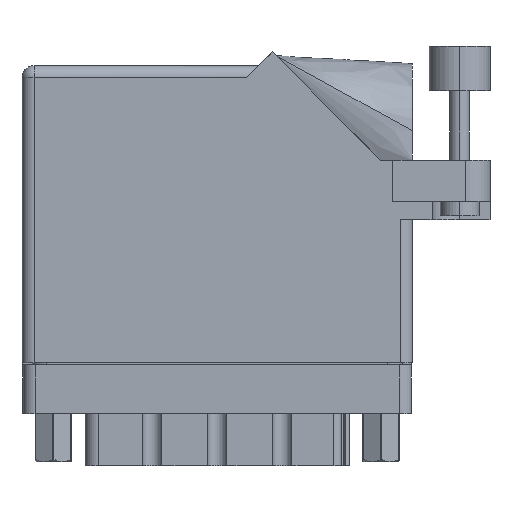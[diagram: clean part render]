
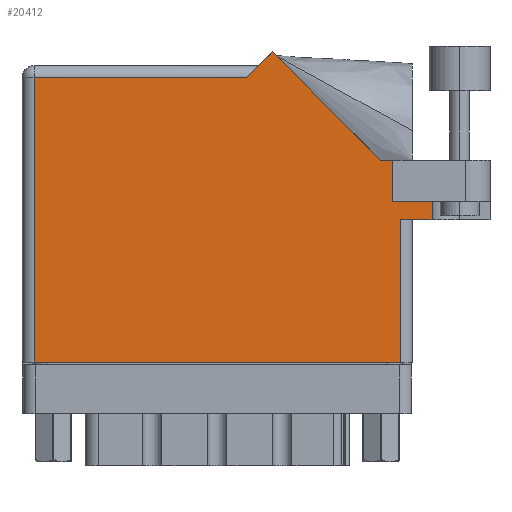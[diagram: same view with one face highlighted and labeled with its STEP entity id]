
A CAD part, front view. The second image highlights one B-rep face of the part: STEP entity #20412.
In plain terms, the highlighted face is planar.
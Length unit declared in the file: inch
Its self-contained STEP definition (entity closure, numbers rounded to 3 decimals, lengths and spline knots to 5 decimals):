
#869 = VECTOR ( 'NONE', #41921, 39.37008 ) ;
#1290 = VERTEX_POINT ( 'NONE', #13275 ) ;
#1875 = VERTEX_POINT ( 'NONE', #25170 ) ;
#2130 = VERTEX_POINT ( 'NONE', #23247 ) ;
#2452 = CARTESIAN_POINT ( 'NONE',  ( 0.062, 0., 0. ) ) ;
#2552 = CARTESIAN_POINT ( 'NONE',  ( 0.062, 1.468, 0. ) ) ;
#2928 = DIRECTION ( 'NONE',  ( -0.707, -0.707, 0. ) ) ;
#4628 = VECTOR ( 'NONE', #13545, 39.37008 ) ;
#5294 = CARTESIAN_POINT ( 'NONE',  ( 1.91, 0.831, 0. ) ) ;
#5372 = LINE ( 'NONE', #5294, #10856 ) ;
#6090 = ORIENTED_EDGE ( 'NONE', *, *, #49748, .T. ) ;
#7015 = CARTESIAN_POINT ( 'NONE',  ( 1.217, 1.53, 0. ) ) ;
#7782 = LINE ( 'NONE', #17917, #24767 ) ;
#8381 = CARTESIAN_POINT ( 'NONE',  ( 1.948, 0., 0. ) ) ;
#9344 = LINE ( 'NONE', #27450, #49462 ) ;
#9447 = DIRECTION ( 'NONE',  ( -1., 0., 0. ) ) ;
#10003 = VECTOR ( 'NONE', #2928, 39.37008 ) ;
#10309 = EDGE_CURVE ( 'NONE', #1290, #27184, #21557, .T. ) ;
#10856 = VECTOR ( 'NONE', #32533, 39.37008 ) ;
#10912 = ORIENTED_EDGE ( 'NONE', *, *, #29694, .T. ) ;
#11082 = VECTOR ( 'NONE', #19312, 39.37008 ) ;
#11657 = DIRECTION ( 'NONE',  ( 0., 1., 0. ) ) ;
#11774 = ORIENTED_EDGE ( 'NONE', *, *, #29884, .T. ) ;
#11809 = VERTEX_POINT ( 'NONE', #26147 ) ;
#13275 = CARTESIAN_POINT ( 'NONE',  ( 1.28771, 1.60071, 0. ) ) ;
#13545 = DIRECTION ( 'NONE',  ( 0., -1., 0. ) ) ;
#13706 = CARTESIAN_POINT ( 'NONE',  ( 1.91, 0.831, 0. ) ) ;
#13804 = VERTEX_POINT ( 'NONE', #38779 ) ;
#15364 = EDGE_CURVE ( 'NONE', #43490, #1875, #5372, .T. ) ;
#16979 = EDGE_LOOP ( 'NONE', ( #19858, #11774, #18190, #32483, #29464, #48066, #10912, #41270, #43193, #6090, #35443 ) ) ;
#17917 = CARTESIAN_POINT ( 'NONE',  ( 0., 1.468, 0. ) ) ;
#18190 = ORIENTED_EDGE ( 'NONE', *, *, #46316, .T. ) ;
#19312 = DIRECTION ( 'NONE',  ( 0., -1., 0. ) ) ;
#19858 = ORIENTED_EDGE ( 'NONE', *, *, #24635, .T. ) ;
#20273 = VERTEX_POINT ( 'NONE', #27319 ) ;
#20412 = ADVANCED_FACE ( 'NONE', ( #48146 ), #47375, .F. ) ;
#20716 = VECTOR ( 'NONE', #22096, 39.37008 ) ;
#21557 = LINE ( 'NONE', #7015, #10003 ) ;
#22037 = CARTESIAN_POINT ( 'NONE',  ( 0., 0., 0. ) ) ;
#22096 = DIRECTION ( 'NONE',  ( -1., 0., 0. ) ) ;
#23247 = CARTESIAN_POINT ( 'NONE',  ( 1.84442, 1.044, 0. ) ) ;
#24066 = DIRECTION ( 'NONE',  ( 0., 0., -1. ) ) ;
#24635 = EDGE_CURVE ( 'NONE', #40682, #27540, #41026, .T. ) ;
#24767 = VECTOR ( 'NONE', #9447, 39.37008 ) ;
#24804 = CARTESIAN_POINT ( 'NONE',  ( 1.84442, 1.044, 0. ) ) ;
#24969 = DIRECTION ( 'NONE',  ( -0.707, 0.707, 0. ) ) ;
#25170 = CARTESIAN_POINT ( 'NONE',  ( 2.1115, 0.831, 0. ) ) ;
#25389 = EDGE_CURVE ( 'NONE', #2130, #1290, #39785, .T. ) ;
#25586 = EDGE_CURVE ( 'NONE', #43490, #13804, #9344, .T. ) ;
#26147 = CARTESIAN_POINT ( 'NONE',  ( 1.948, 0.737, 0. ) ) ;
#26801 = LINE ( 'NONE', #37617, #20716 ) ;
#27184 = VERTEX_POINT ( 'NONE', #30011 ) ;
#27319 = CARTESIAN_POINT ( 'NONE',  ( 2.1115, 0.737, 0. ) ) ;
#27450 = CARTESIAN_POINT ( 'NONE',  ( 1.91, 0.831, 0. ) ) ;
#27540 = VERTEX_POINT ( 'NONE', #8381 ) ;
#29464 = ORIENTED_EDGE ( 'NONE', *, *, #15364, .F. ) ;
#29694 = EDGE_CURVE ( 'NONE', #13804, #2130, #26801, .T. ) ;
#29884 = EDGE_CURVE ( 'NONE', #27540, #11809, #43830, .T. ) ;
#30011 = CARTESIAN_POINT ( 'NONE',  ( 1.155, 1.468, 0. ) ) ;
#30642 = AXIS2_PLACEMENT_3D ( 'NONE', #35525, #24066, #47543 ) ;
#32483 = ORIENTED_EDGE ( 'NONE', *, *, #47893, .F. ) ;
#32533 = DIRECTION ( 'NONE',  ( 1., 0., 0. ) ) ;
#32699 = DIRECTION ( 'NONE',  ( 1., 0., 0. ) ) ;
#33525 = VECTOR ( 'NONE', #50132, 39.37008 ) ;
#34245 = LINE ( 'NONE', #2452, #11082 ) ;
#34546 = CARTESIAN_POINT ( 'NONE',  ( 1.948, 0.737, 0. ) ) ;
#35443 = ORIENTED_EDGE ( 'NONE', *, *, #43655, .T. ) ;
#35525 = CARTESIAN_POINT ( 'NONE',  ( 0., 1.53, 0. ) ) ;
#37613 = VECTOR ( 'NONE', #32699, 39.37008 ) ;
#37617 = CARTESIAN_POINT ( 'NONE',  ( 2.41, 1.044, 0. ) ) ;
#38779 = CARTESIAN_POINT ( 'NONE',  ( 1.91, 1.044, 0. ) ) ;
#39785 = LINE ( 'NONE', #24804, #48880 ) ;
#40491 = CARTESIAN_POINT ( 'NONE',  ( 2.01, 0.737, 0. ) ) ;
#40578 = CARTESIAN_POINT ( 'NONE',  ( 2.1115, 1.16177, 0. ) ) ;
#40682 = VERTEX_POINT ( 'NONE', #45259 ) ;
#41026 = LINE ( 'NONE', #22037, #869 ) ;
#41270 = ORIENTED_EDGE ( 'NONE', *, *, #25389, .T. ) ;
#41921 = DIRECTION ( 'NONE',  ( 1., 0., 0. ) ) ;
#43193 = ORIENTED_EDGE ( 'NONE', *, *, #10309, .T. ) ;
#43490 = VERTEX_POINT ( 'NONE', #13706 ) ;
#43655 = EDGE_CURVE ( 'NONE', #48642, #40682, #34245, .T. ) ;
#43830 = LINE ( 'NONE', #34546, #33525 ) ;
#44805 = LINE ( 'NONE', #40578, #4628 ) ;
#45259 = CARTESIAN_POINT ( 'NONE',  ( 0.062, 0., 0. ) ) ;
#46316 = EDGE_CURVE ( 'NONE', #11809, #20273, #48498, .T. ) ;
#47375 = PLANE ( 'NONE',  #30642 ) ;
#47543 = DIRECTION ( 'NONE',  ( -1., 0., 0. ) ) ;
#47893 = EDGE_CURVE ( 'NONE', #1875, #20273, #44805, .T. ) ;
#48066 = ORIENTED_EDGE ( 'NONE', *, *, #25586, .T. ) ;
#48146 = FACE_OUTER_BOUND ( 'NONE', #16979, .T. ) ;
#48498 = LINE ( 'NONE', #40491, #37613 ) ;
#48642 = VERTEX_POINT ( 'NONE', #2552 ) ;
#48880 = VECTOR ( 'NONE', #24969, 39.37008 ) ;
#49462 = VECTOR ( 'NONE', #11657, 39.37008 ) ;
#49748 = EDGE_CURVE ( 'NONE', #27184, #48642, #7782, .T. ) ;
#50132 = DIRECTION ( 'NONE',  ( 0., 1., 0. ) ) ;
